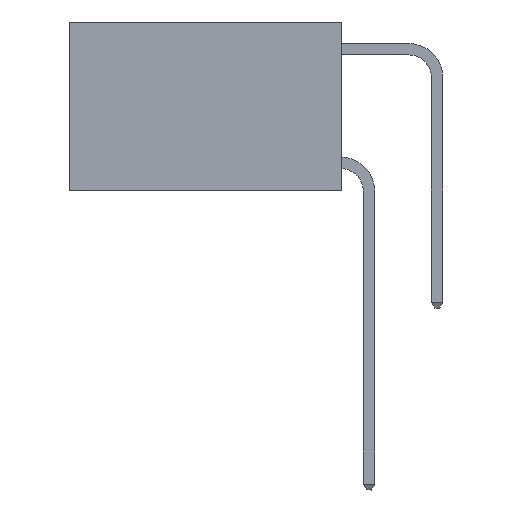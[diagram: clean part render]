
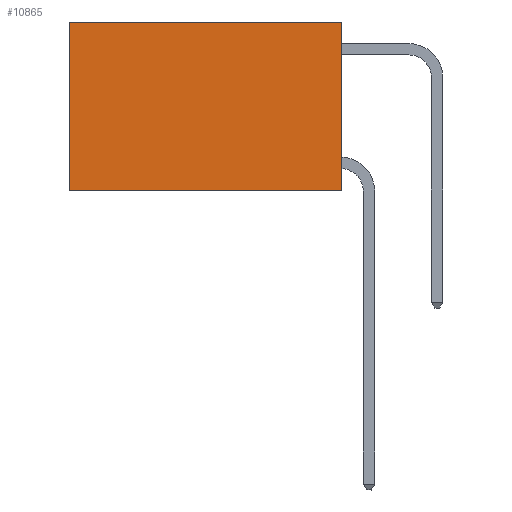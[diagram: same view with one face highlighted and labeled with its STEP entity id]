
A CAD part, left-side view. The second image highlights one B-rep face of the part: STEP entity #10865.
In plain terms, the highlighted planar face has unit normal (-1, 0, 0).
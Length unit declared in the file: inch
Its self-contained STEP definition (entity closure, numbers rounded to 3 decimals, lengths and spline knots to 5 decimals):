
#1287 = EDGE_LOOP ( 'NONE', ( #5442, #9108, #15806, #3196 ) ) ;
#1334 = CARTESIAN_POINT ( 'NONE',  ( 0.2625, 0., 0. ) ) ;
#1351 = LINE ( 'NONE', #11693, #17927 ) ;
#1698 = DIRECTION ( 'NONE',  ( 0., 0., -1. ) ) ;
#1901 = VECTOR ( 'NONE', #1698, 39.37008 ) ;
#2014 = PLANE ( 'NONE',  #6031 ) ;
#3159 = VECTOR ( 'NONE', #16604, 39.37008 ) ;
#3196 = ORIENTED_EDGE ( 'NONE', *, *, #9990, .T. ) ;
#3433 = VERTEX_POINT ( 'NONE', #20595 ) ;
#4416 = VERTEX_POINT ( 'NONE', #13423 ) ;
#5270 = DIRECTION ( 'NONE',  ( 0., 0., -1. ) ) ;
#5385 = CARTESIAN_POINT ( 'NONE',  ( 0.2625, 0.6, 0. ) ) ;
#5388 = CARTESIAN_POINT ( 'NONE',  ( 0.2625, 0., 0. ) ) ;
#5442 = ORIENTED_EDGE ( 'NONE', *, *, #7414, .T. ) ;
#5886 = FACE_OUTER_BOUND ( 'NONE', #1287, .T. ) ;
#6031 = AXIS2_PLACEMENT_3D ( 'NONE', #5388, #16561, #6996 ) ;
#6996 = DIRECTION ( 'NONE',  ( 0., 0., -1. ) ) ;
#7044 = CARTESIAN_POINT ( 'NONE',  ( 0.2625, 0., -0.37 ) ) ;
#7414 = EDGE_CURVE ( 'NONE', #11456, #3433, #18452, .T. ) ;
#7961 = LINE ( 'NONE', #1334, #16405 ) ;
#8248 = EDGE_CURVE ( 'NONE', #4416, #11247, #1351, .T. ) ;
#9108 = ORIENTED_EDGE ( 'NONE', *, *, #13983, .F. ) ;
#9843 = CARTESIAN_POINT ( 'NONE',  ( 0.2625, 0.6, 0. ) ) ;
#9885 = CARTESIAN_POINT ( 'NONE',  ( 0.2625, 0., -0.37 ) ) ;
#9990 = EDGE_CURVE ( 'NONE', #4416, #11456, #7961, .T. ) ;
#10865 = ADVANCED_FACE ( 'NONE', ( #5886 ), #2014, .F. ) ;
#11247 = VERTEX_POINT ( 'NONE', #9885 ) ;
#11456 = VERTEX_POINT ( 'NONE', #5385 ) ;
#11693 = CARTESIAN_POINT ( 'NONE',  ( 0.2625, 0., 0. ) ) ;
#13423 = CARTESIAN_POINT ( 'NONE',  ( 0.2625, 0., 0. ) ) ;
#13983 = EDGE_CURVE ( 'NONE', #11247, #3433, #15478, .T. ) ;
#15478 = LINE ( 'NONE', #7044, #3159 ) ;
#15806 = ORIENTED_EDGE ( 'NONE', *, *, #8248, .F. ) ;
#16405 = VECTOR ( 'NONE', #18898, 39.37008 ) ;
#16561 = DIRECTION ( 'NONE',  ( 1., 0., 0. ) ) ;
#16604 = DIRECTION ( 'NONE',  ( 0., 1., 0. ) ) ;
#17927 = VECTOR ( 'NONE', #5270, 39.37008 ) ;
#18452 = LINE ( 'NONE', #9843, #1901 ) ;
#18898 = DIRECTION ( 'NONE',  ( 0., 1., 0. ) ) ;
#20595 = CARTESIAN_POINT ( 'NONE',  ( 0.2625, 0.6, -0.37 ) ) ;
